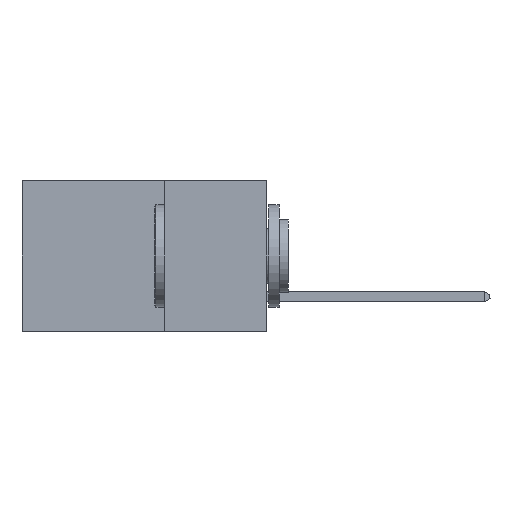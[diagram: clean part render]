
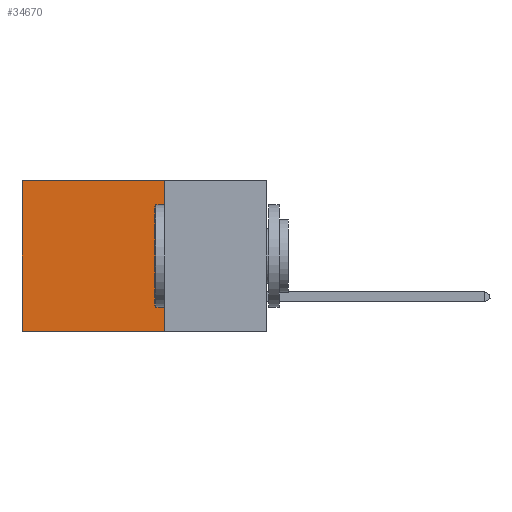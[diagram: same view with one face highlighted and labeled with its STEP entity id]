
A CAD part, left-side view. The second image highlights one B-rep face of the part: STEP entity #34670.
In plain terms, the highlighted planar face has unit normal (-1, 0, 0).
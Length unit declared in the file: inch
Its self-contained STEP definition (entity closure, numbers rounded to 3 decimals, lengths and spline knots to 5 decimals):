
#165 = CARTESIAN_POINT ( 'NONE',  ( 0.2875, 0.6, 0. ) ) ;
#171 = DIRECTION ( 'NONE',  ( 0., 1., 0. ) ) ;
#2618 = CARTESIAN_POINT ( 'NONE',  ( 0.2875, 0.25, 0. ) ) ;
#5353 = VECTOR ( 'NONE', #171, 39.37008 ) ;
#6053 = FACE_OUTER_BOUND ( 'NONE', #42949, .T. ) ;
#6230 = LINE ( 'NONE', #165, #41452 ) ;
#6866 = DIRECTION ( 'NONE',  ( 0., 0., -1. ) ) ;
#9827 = EDGE_CURVE ( 'NONE', #19230, #46524, #26050, .T. ) ;
#12667 = CARTESIAN_POINT ( 'NONE',  ( 0.2875, 0.25, 0. ) ) ;
#12706 = DIRECTION ( 'NONE',  ( 0., 0., -1. ) ) ;
#12735 = DIRECTION ( 'NONE',  ( 0., 0., -1. ) ) ;
#14680 = VECTOR ( 'NONE', #27485, 39.37008 ) ;
#14846 = EDGE_CURVE ( 'NONE', #19230, #43419, #30249, .T. ) ;
#15610 = CARTESIAN_POINT ( 'NONE',  ( 0.2875, 0.25, -0.37 ) ) ;
#16500 = VERTEX_POINT ( 'NONE', #21130 ) ;
#19230 = VERTEX_POINT ( 'NONE', #27346 ) ;
#19959 = ORIENTED_EDGE ( 'NONE', *, *, #44212, .F. ) ;
#21130 = CARTESIAN_POINT ( 'NONE',  ( 0.2875, 0.6, -0.37 ) ) ;
#21361 = PLANE ( 'NONE',  #42687 ) ;
#22801 = ORIENTED_EDGE ( 'NONE', *, *, #9827, .T. ) ;
#24484 = ORIENTED_EDGE ( 'NONE', *, *, #32413, .T. ) ;
#24515 = CARTESIAN_POINT ( 'NONE',  ( 0.2875, 0.6, 0. ) ) ;
#25026 = DIRECTION ( 'NONE',  ( 1., 0., 0. ) ) ;
#26050 = LINE ( 'NONE', #12667, #14680 ) ;
#27346 = CARTESIAN_POINT ( 'NONE',  ( 0.2875, 0.25, 0. ) ) ;
#27485 = DIRECTION ( 'NONE',  ( 0., 1., 0. ) ) ;
#30249 = LINE ( 'NONE', #2618, #32551 ) ;
#32413 = EDGE_CURVE ( 'NONE', #46524, #16500, #6230, .T. ) ;
#32551 = VECTOR ( 'NONE', #12735, 39.37008 ) ;
#34670 = ADVANCED_FACE ( 'NONE', ( #6053 ), #21361, .F. ) ;
#37159 = LINE ( 'NONE', #44326, #5353 ) ;
#38056 = ORIENTED_EDGE ( 'NONE', *, *, #14846, .F. ) ;
#39617 = CARTESIAN_POINT ( 'NONE',  ( 0.2875, 0.25, 0. ) ) ;
#41452 = VECTOR ( 'NONE', #12706, 39.37008 ) ;
#42687 = AXIS2_PLACEMENT_3D ( 'NONE', #39617, #25026, #6866 ) ;
#42949 = EDGE_LOOP ( 'NONE', ( #24484, #19959, #38056, #22801 ) ) ;
#43419 = VERTEX_POINT ( 'NONE', #15610 ) ;
#44212 = EDGE_CURVE ( 'NONE', #43419, #16500, #37159, .T. ) ;
#44326 = CARTESIAN_POINT ( 'NONE',  ( 0.2875, 0.25, -0.37 ) ) ;
#46524 = VERTEX_POINT ( 'NONE', #24515 ) ;
